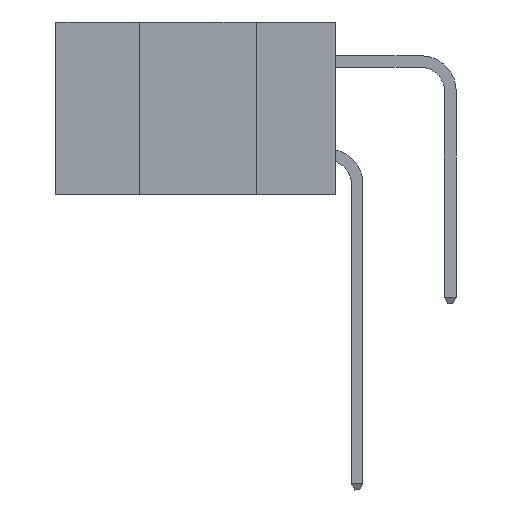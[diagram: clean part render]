
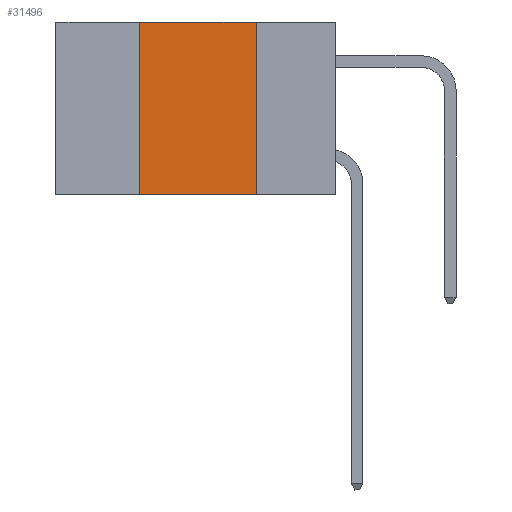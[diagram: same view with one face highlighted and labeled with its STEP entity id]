
A CAD part, left-side view. The second image highlights one B-rep face of the part: STEP entity #31496.
In plain terms, the highlighted planar face has unit normal (-1, 0, 0).
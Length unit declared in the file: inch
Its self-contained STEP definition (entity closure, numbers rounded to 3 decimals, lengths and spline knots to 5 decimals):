
#268 = VECTOR ( 'NONE', #24384, 39.37008 ) ;
#3768 = VERTEX_POINT ( 'NONE', #8705 ) ;
#4595 = DIRECTION ( 'NONE',  ( 1., 0., 0. ) ) ;
#4709 = VECTOR ( 'NONE', #30192, 39.37008 ) ;
#5419 = ORIENTED_EDGE ( 'NONE', *, *, #26216, .F. ) ;
#7823 = DIRECTION ( 'NONE',  ( 0., 0., -1. ) ) ;
#8686 = ORIENTED_EDGE ( 'NONE', *, *, #16908, .F. ) ;
#8705 = CARTESIAN_POINT ( 'NONE',  ( 0., 0.17, 0. ) ) ;
#9025 = VECTOR ( 'NONE', #21465, 39.37008 ) ;
#9848 = LINE ( 'NONE', #34120, #268 ) ;
#10543 = VERTEX_POINT ( 'NONE', #28955 ) ;
#11077 = CARTESIAN_POINT ( 'NONE',  ( 0., 0.17, 0. ) ) ;
#14783 = ORIENTED_EDGE ( 'NONE', *, *, #35409, .T. ) ;
#16908 = EDGE_CURVE ( 'NONE', #35841, #3768, #9848, .T. ) ;
#20117 = EDGE_LOOP ( 'NONE', ( #26176, #8686, #5419, #14783 ) ) ;
#21465 = DIRECTION ( 'NONE',  ( 0., -1., 0. ) ) ;
#21791 = VECTOR ( 'NONE', #29497, 39.37008 ) ;
#24384 = DIRECTION ( 'NONE',  ( 0., -1., 0. ) ) ;
#25855 = LINE ( 'NONE', #37315, #9025 ) ;
#26176 = ORIENTED_EDGE ( 'NONE', *, *, #29006, .F. ) ;
#26216 = EDGE_CURVE ( 'NONE', #29482, #35841, #33238, .T. ) ;
#27505 = AXIS2_PLACEMENT_3D ( 'NONE', #29827, #4595, #7823 ) ;
#28955 = CARTESIAN_POINT ( 'NONE',  ( 0., 0.17, -0.37 ) ) ;
#29006 = EDGE_CURVE ( 'NONE', #3768, #10543, #37493, .T. ) ;
#29349 = CARTESIAN_POINT ( 'NONE',  ( 0., 0.42, 0. ) ) ;
#29482 = VERTEX_POINT ( 'NONE', #32352 ) ;
#29497 = DIRECTION ( 'NONE',  ( 0., 0., 1. ) ) ;
#29827 = CARTESIAN_POINT ( 'NONE',  ( 0., 0.6, 0. ) ) ;
#30171 = CARTESIAN_POINT ( 'NONE',  ( 0., 0.42, 0. ) ) ;
#30192 = DIRECTION ( 'NONE',  ( 0., 0., -1. ) ) ;
#30627 = FACE_OUTER_BOUND ( 'NONE', #20117, .T. ) ;
#31496 = ADVANCED_FACE ( 'NONE', ( #30627 ), #36256, .F. ) ;
#32352 = CARTESIAN_POINT ( 'NONE',  ( 0., 0.42, -0.37 ) ) ;
#33238 = LINE ( 'NONE', #29349, #21791 ) ;
#34120 = CARTESIAN_POINT ( 'NONE',  ( 0., 0.6, 0. ) ) ;
#35409 = EDGE_CURVE ( 'NONE', #29482, #10543, #25855, .T. ) ;
#35841 = VERTEX_POINT ( 'NONE', #30171 ) ;
#36256 = PLANE ( 'NONE',  #27505 ) ;
#37315 = CARTESIAN_POINT ( 'NONE',  ( 0., 0.6, -0.37 ) ) ;
#37493 = LINE ( 'NONE', #11077, #4709 ) ;
